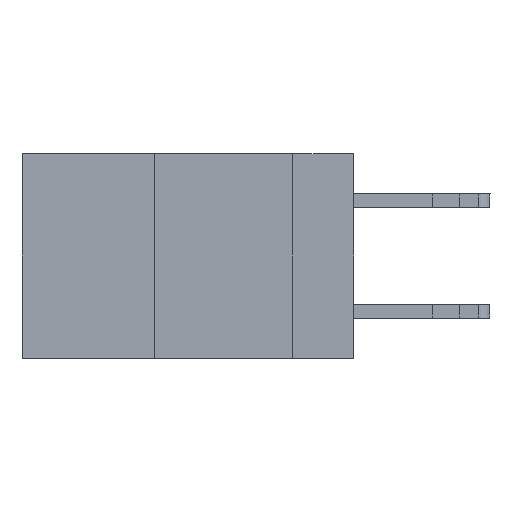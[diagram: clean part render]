
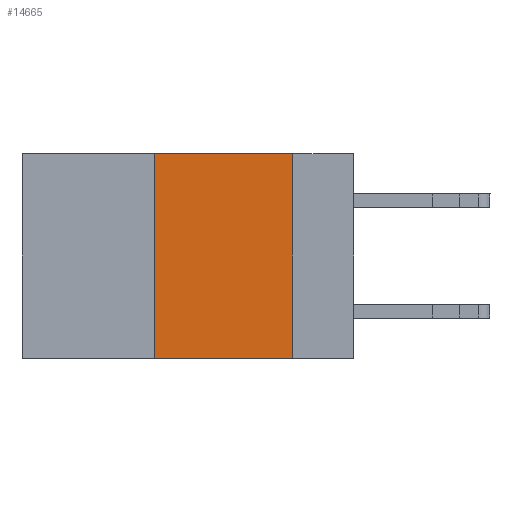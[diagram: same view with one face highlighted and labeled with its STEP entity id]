
A CAD part, left-side view. The second image highlights one B-rep face of the part: STEP entity #14665.
In plain terms, the highlighted planar face has unit normal (-1, 0, 0).
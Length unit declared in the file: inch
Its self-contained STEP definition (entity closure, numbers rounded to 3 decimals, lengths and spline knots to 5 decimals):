
#625 = DIRECTION ( 'NONE',  ( 0., -1., 0. ) ) ;
#929 = DIRECTION ( 'NONE',  ( 0., 0., -1. ) ) ;
#1089 = PLANE ( 'NONE',  #8254 ) ;
#1637 = VERTEX_POINT ( 'NONE', #5522 ) ;
#2373 = VECTOR ( 'NONE', #10291, 39.37008 ) ;
#2736 = CARTESIAN_POINT ( 'NONE',  ( 0., 0.6, 0. ) ) ;
#2953 = ORIENTED_EDGE ( 'NONE', *, *, #11245, .F. ) ;
#2965 = DIRECTION ( 'NONE',  ( 0., 0., 1. ) ) ;
#3436 = CARTESIAN_POINT ( 'NONE',  ( 0., 0.11, -0.37 ) ) ;
#4337 = EDGE_CURVE ( 'NONE', #1637, #9239, #11602, .T. ) ;
#4807 = CARTESIAN_POINT ( 'NONE',  ( 0., 0.6, -0.37 ) ) ;
#5211 = EDGE_LOOP ( 'NONE', ( #7539, #11434, #2953, #12229 ) ) ;
#5522 = CARTESIAN_POINT ( 'NONE',  ( 0., 0.11, 0. ) ) ;
#6210 = FACE_OUTER_BOUND ( 'NONE', #5211, .T. ) ;
#7505 = DIRECTION ( 'NONE',  ( 1., 0., 0. ) ) ;
#7539 = ORIENTED_EDGE ( 'NONE', *, *, #4337, .F. ) ;
#8254 = AXIS2_PLACEMENT_3D ( 'NONE', #17019, #7505, #11511 ) ;
#8979 = VECTOR ( 'NONE', #929, 39.37008 ) ;
#9235 = LINE ( 'NONE', #2736, #2373 ) ;
#9239 = VERTEX_POINT ( 'NONE', #3436 ) ;
#9603 = VECTOR ( 'NONE', #2965, 39.37008 ) ;
#9826 = LINE ( 'NONE', #4807, #15704 ) ;
#10291 = DIRECTION ( 'NONE',  ( 0., -1., 0. ) ) ;
#10504 = CARTESIAN_POINT ( 'NONE',  ( 0., 0.36, 0. ) ) ;
#10936 = LINE ( 'NONE', #13631, #9603 ) ;
#10999 = EDGE_CURVE ( 'NONE', #11183, #9239, #9826, .T. ) ;
#11183 = VERTEX_POINT ( 'NONE', #15560 ) ;
#11245 = EDGE_CURVE ( 'NONE', #11183, #15578, #10936, .T. ) ;
#11434 = ORIENTED_EDGE ( 'NONE', *, *, #12139, .F. ) ;
#11511 = DIRECTION ( 'NONE',  ( 0., 0., -1. ) ) ;
#11519 = CARTESIAN_POINT ( 'NONE',  ( 0., 0.11, 0. ) ) ;
#11602 = LINE ( 'NONE', #11519, #8979 ) ;
#12139 = EDGE_CURVE ( 'NONE', #15578, #1637, #9235, .T. ) ;
#12229 = ORIENTED_EDGE ( 'NONE', *, *, #10999, .T. ) ;
#13631 = CARTESIAN_POINT ( 'NONE',  ( 0., 0.36, 0. ) ) ;
#14665 = ADVANCED_FACE ( 'NONE', ( #6210 ), #1089, .F. ) ;
#15560 = CARTESIAN_POINT ( 'NONE',  ( 0., 0.36, -0.37 ) ) ;
#15578 = VERTEX_POINT ( 'NONE', #10504 ) ;
#15704 = VECTOR ( 'NONE', #625, 39.37008 ) ;
#17019 = CARTESIAN_POINT ( 'NONE',  ( 0., 0.6, 0. ) ) ;
